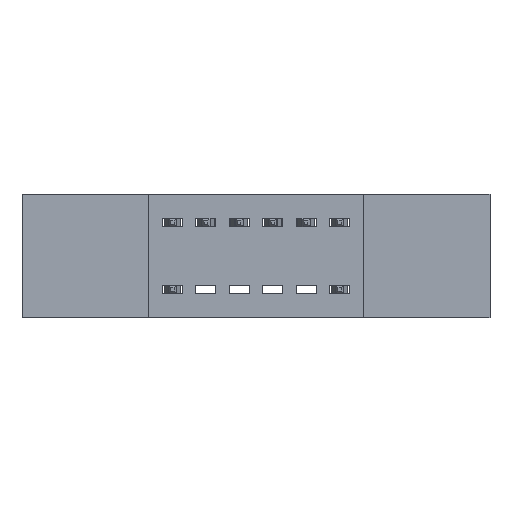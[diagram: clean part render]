
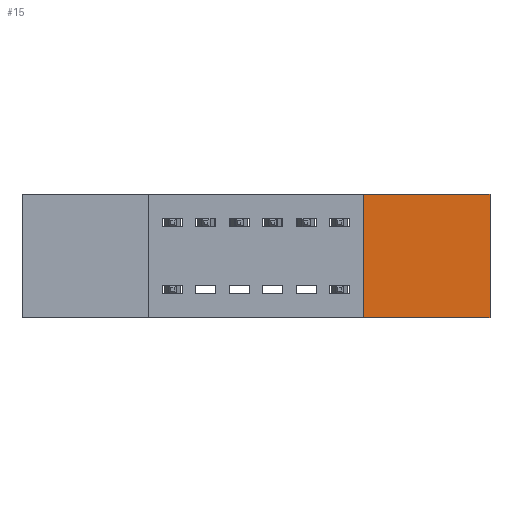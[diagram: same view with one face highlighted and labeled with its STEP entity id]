
A CAD part, front view. The second image highlights one B-rep face of the part: STEP entity #15.
In plain terms, the highlighted planar face has unit normal (0, -1, 0).
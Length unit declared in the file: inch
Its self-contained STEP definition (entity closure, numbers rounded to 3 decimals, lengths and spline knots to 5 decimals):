
#15 = ADVANCED_FACE ( 'NONE', ( #4442 ), #2358, .T. ) ;
#246 = CARTESIAN_POINT ( 'NONE',  ( 1.4, 0., 0. ) ) ;
#591 = CARTESIAN_POINT ( 'NONE',  ( 0., 0., 0. ) ) ;
#616 = ORIENTED_EDGE ( 'NONE', *, *, #6572, .F. ) ;
#620 = CARTESIAN_POINT ( 'NONE',  ( 1.023, 0., -0.37 ) ) ;
#670 = LINE ( 'NONE', #3441, #5685 ) ;
#1264 = VECTOR ( 'NONE', #1356, 39.37008 ) ;
#1356 = DIRECTION ( 'NONE',  ( -1., 0., 0. ) ) ;
#1541 = DIRECTION ( 'NONE',  ( 0., 0., -1. ) ) ;
#1663 = VERTEX_POINT ( 'NONE', #6422 ) ;
#2262 = EDGE_LOOP ( 'NONE', ( #616, #3709, #2823, #5774 ) ) ;
#2358 = PLANE ( 'NONE',  #8038 ) ;
#2823 = ORIENTED_EDGE ( 'NONE', *, *, #3108, .F. ) ;
#3108 = EDGE_CURVE ( 'NONE', #6904, #1663, #670, .T. ) ;
#3395 = DIRECTION ( 'NONE',  ( 0., 0., -1. ) ) ;
#3441 = CARTESIAN_POINT ( 'NONE',  ( 1.4, 0., 0. ) ) ;
#3709 = ORIENTED_EDGE ( 'NONE', *, *, #5740, .F. ) ;
#4192 = VECTOR ( 'NONE', #6876, 39.37008 ) ;
#4406 = VECTOR ( 'NONE', #6985, 39.37008 ) ;
#4442 = FACE_OUTER_BOUND ( 'NONE', #2262, .T. ) ;
#4488 = CARTESIAN_POINT ( 'NONE',  ( 0., 0., -0.37 ) ) ;
#4570 = CARTESIAN_POINT ( 'NONE',  ( 1.023, 0., -0.37 ) ) ;
#4858 = LINE ( 'NONE', #4488, #1264 ) ;
#5685 = VECTOR ( 'NONE', #1541, 39.37008 ) ;
#5740 = EDGE_CURVE ( 'NONE', #1663, #6432, #4858, .T. ) ;
#5774 = ORIENTED_EDGE ( 'NONE', *, *, #7019, .F. ) ;
#6009 = LINE ( 'NONE', #4570, #4192 ) ;
#6422 = CARTESIAN_POINT ( 'NONE',  ( 1.4, 0., -0.37 ) ) ;
#6432 = VERTEX_POINT ( 'NONE', #620 ) ;
#6572 = EDGE_CURVE ( 'NONE', #6432, #7566, #6009, .T. ) ;
#6876 = DIRECTION ( 'NONE',  ( 0., 0., 1. ) ) ;
#6904 = VERTEX_POINT ( 'NONE', #246 ) ;
#6985 = DIRECTION ( 'NONE',  ( 1., 0., 0. ) ) ;
#7019 = EDGE_CURVE ( 'NONE', #7566, #6904, #7973, .T. ) ;
#7054 = CARTESIAN_POINT ( 'NONE',  ( 1.023, 0., 0. ) ) ;
#7498 = CARTESIAN_POINT ( 'NONE',  ( 0., 0., -0.37 ) ) ;
#7566 = VERTEX_POINT ( 'NONE', #7054 ) ;
#7973 = LINE ( 'NONE', #591, #4406 ) ;
#8038 = AXIS2_PLACEMENT_3D ( 'NONE', #7498, #8124, #3395 ) ;
#8124 = DIRECTION ( 'NONE',  ( 0., -1., 0. ) ) ;
